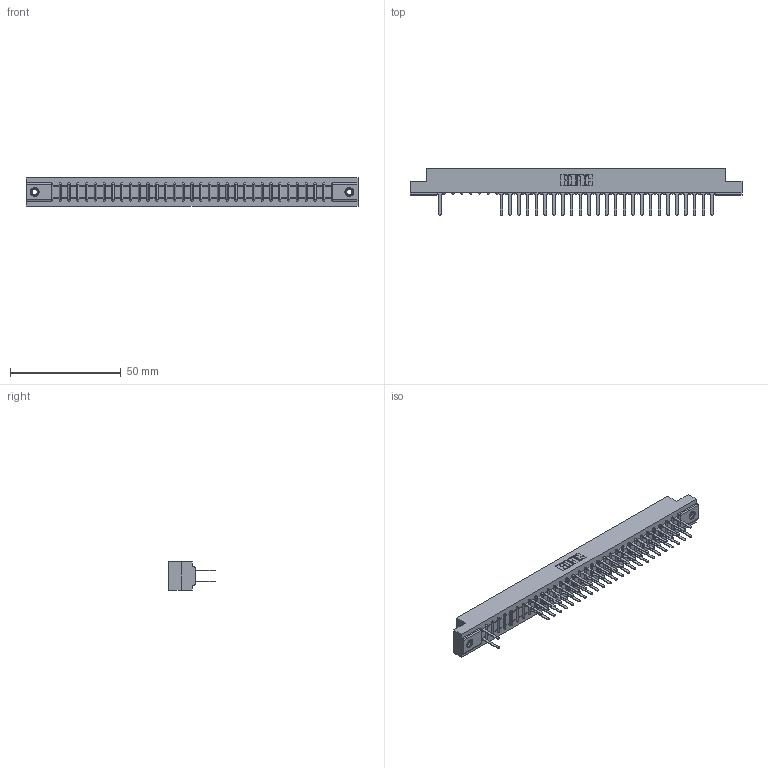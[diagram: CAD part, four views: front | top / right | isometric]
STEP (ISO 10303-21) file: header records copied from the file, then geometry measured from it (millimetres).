
FILE_DESCRIPTION (( 'STEP AP203' ), '1' );
FILE_NAME ('307-064-522-207.STEP', '2018-08-06T10:00:54', ( '' ), ( '' ), 'SwSTEP 2.0', 'SolidWorks 2016', '' );
FILE_SCHEMA (( 'CONFIG_CONTROL_DESIGN' ));
Length unit declared in the file: inch
Products named in the file (4): 307 Part_.156 Dia Mounting Holes; 307-290-001_522; 345-250-001_345-250-005-103; 307-064-522-207
Assembly tree (54 placements, depth 2):
  307-064-522-207
    307 Part_.156 Dia Mounting Holes
    307-290-001_522  x51
    345-250-001_345-250-005-103  x2
Bounding box: 149.81 x 21.11 x 12.7 mm (x, y, z)
Volume: 15787.6 mm3; surface area: 18599.4 mm2
Topology: 54 solids, 54 shells, 2687 faces, 7505 edges, 4838 vertices
Faces by surface type: plane 1761, cylinder 844, sphere 66, cone 12, torus 4
Entity records: 30427 total; most frequent: CARTESIAN_POINT 5018, ORIENTED_EDGE 4978, DIRECTION 4915, EDGE_CURVE 2489, VECTOR 1905, LINE 1905, VERTEX_POINT 1608, AXIS2_PLACEMENT_3D 1505
